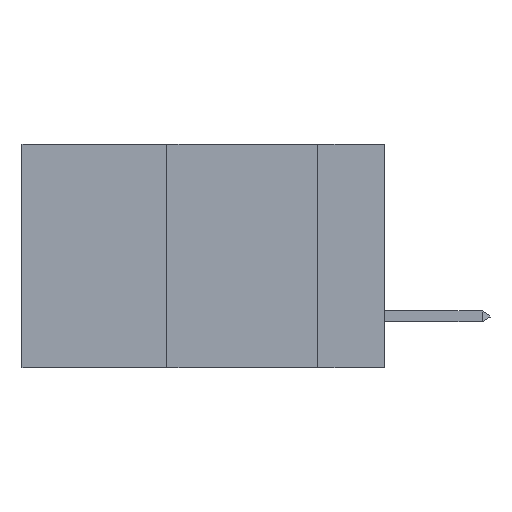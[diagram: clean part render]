
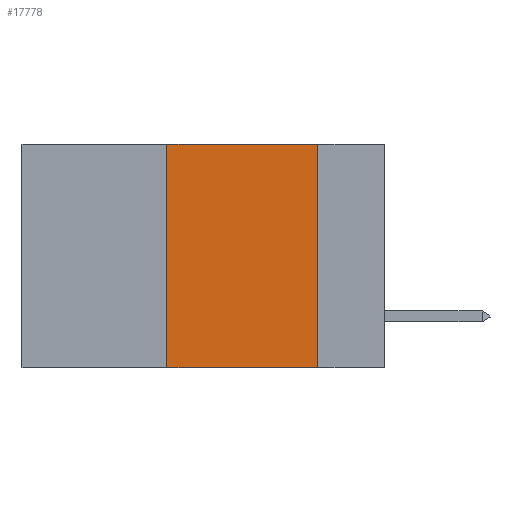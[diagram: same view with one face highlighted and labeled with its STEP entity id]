
A CAD part, left-side view. The second image highlights one B-rep face of the part: STEP entity #17778.
In plain terms, the highlighted planar face has unit normal (-1, 0, 0).
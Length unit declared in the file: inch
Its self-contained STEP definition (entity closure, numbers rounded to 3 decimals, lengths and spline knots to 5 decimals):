
#326 = ORIENTED_EDGE ( 'NONE', *, *, #6067, .F. ) ;
#1044 = ORIENTED_EDGE ( 'NONE', *, *, #3288, .T. ) ;
#1960 = EDGE_LOOP ( 'NONE', ( #326, #4065, #16639, #1044 ) ) ;
#2147 = VECTOR ( 'NONE', #11376, 39.37008 ) ;
#2771 = CARTESIAN_POINT ( 'NONE',  ( 0., 0.36, -0.37 ) ) ;
#2843 = DIRECTION ( 'NONE',  ( 0., 0., -1. ) ) ;
#2985 = CARTESIAN_POINT ( 'NONE',  ( 0., 0.6, 0. ) ) ;
#3031 = LINE ( 'NONE', #12396, #20438 ) ;
#3288 = EDGE_CURVE ( 'NONE', #11511, #5164, #8159, .T. ) ;
#3456 = CARTESIAN_POINT ( 'NONE',  ( 0., 0.11, -0.37 ) ) ;
#4065 = ORIENTED_EDGE ( 'NONE', *, *, #10051, .F. ) ;
#5164 = VERTEX_POINT ( 'NONE', #3456 ) ;
#6067 = EDGE_CURVE ( 'NONE', #20861, #5164, #6672, .T. ) ;
#6332 = CARTESIAN_POINT ( 'NONE',  ( 0., 0.11, 0. ) ) ;
#6672 = LINE ( 'NONE', #6332, #2147 ) ;
#8159 = LINE ( 'NONE', #12214, #10217 ) ;
#9225 = DIRECTION ( 'NONE',  ( 0., 0., 1. ) ) ;
#9446 = PLANE ( 'NONE',  #15632 ) ;
#9574 = VECTOR ( 'NONE', #9225, 39.37008 ) ;
#9915 = CARTESIAN_POINT ( 'NONE',  ( 0., 0.36, 0. ) ) ;
#10051 = EDGE_CURVE ( 'NONE', #11073, #20861, #3031, .T. ) ;
#10217 = VECTOR ( 'NONE', #13764, 39.37008 ) ;
#11073 = VERTEX_POINT ( 'NONE', #9915 ) ;
#11376 = DIRECTION ( 'NONE',  ( 0., 0., -1. ) ) ;
#11511 = VERTEX_POINT ( 'NONE', #2771 ) ;
#11743 = EDGE_CURVE ( 'NONE', #11511, #11073, #20914, .T. ) ;
#12214 = CARTESIAN_POINT ( 'NONE',  ( 0., 0.6, -0.37 ) ) ;
#12396 = CARTESIAN_POINT ( 'NONE',  ( 0., 0.6, 0. ) ) ;
#13764 = DIRECTION ( 'NONE',  ( 0., -1., 0. ) ) ;
#15632 = AXIS2_PLACEMENT_3D ( 'NONE', #2985, #18209, #2843 ) ;
#16295 = CARTESIAN_POINT ( 'NONE',  ( 0., 0.11, 0. ) ) ;
#16639 = ORIENTED_EDGE ( 'NONE', *, *, #11743, .F. ) ;
#17778 = ADVANCED_FACE ( 'NONE', ( #19814 ), #9446, .F. ) ;
#18209 = DIRECTION ( 'NONE',  ( 1., 0., 0. ) ) ;
#19018 = DIRECTION ( 'NONE',  ( 0., -1., 0. ) ) ;
#19814 = FACE_OUTER_BOUND ( 'NONE', #1960, .T. ) ;
#20438 = VECTOR ( 'NONE', #19018, 39.37008 ) ;
#20861 = VERTEX_POINT ( 'NONE', #16295 ) ;
#20863 = CARTESIAN_POINT ( 'NONE',  ( 0., 0.36, 0. ) ) ;
#20914 = LINE ( 'NONE', #20863, #9574 ) ;
